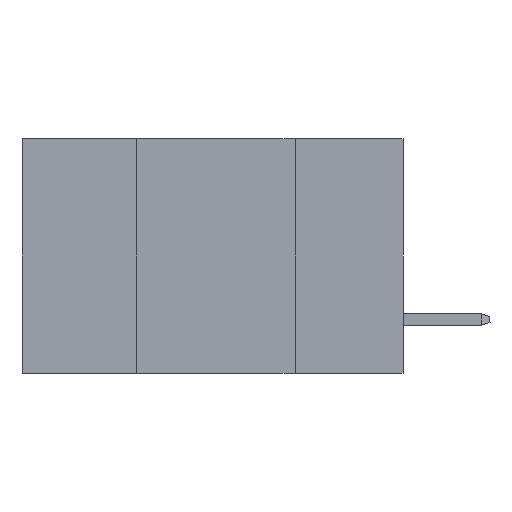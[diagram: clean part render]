
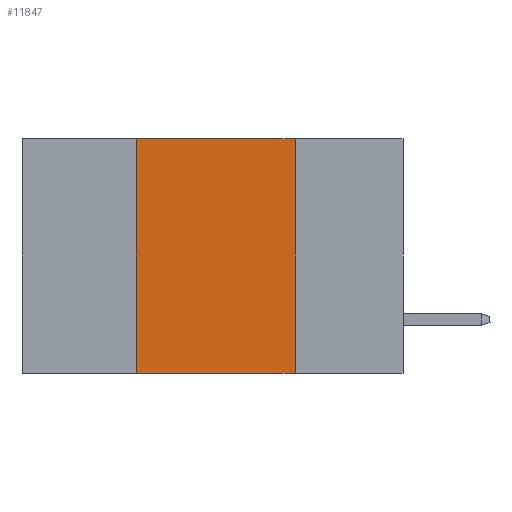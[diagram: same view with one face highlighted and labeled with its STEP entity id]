
A CAD part, left-side view. The second image highlights one B-rep face of the part: STEP entity #11847.
In plain terms, the highlighted planar face has unit normal (-1, 0, 0).
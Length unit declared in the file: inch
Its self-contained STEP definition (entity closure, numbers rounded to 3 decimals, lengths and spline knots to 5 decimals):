
#142 = DIRECTION ( 'NONE',  ( 1., 0., 0. ) ) ;
#355 = ORIENTED_EDGE ( 'NONE', *, *, #10931, .F. ) ;
#928 = EDGE_CURVE ( 'NONE', #3496, #2438, #9647, .T. ) ;
#961 = DIRECTION ( 'NONE',  ( 0., 0., -1. ) ) ;
#2438 = VERTEX_POINT ( 'NONE', #13421 ) ;
#2498 = EDGE_CURVE ( 'NONE', #3496, #14321, #9845, .T. ) ;
#3439 = DIRECTION ( 'NONE',  ( 0., 0., 1. ) ) ;
#3496 = VERTEX_POINT ( 'NONE', #16037 ) ;
#4150 = VECTOR ( 'NONE', #961, 39.37008 ) ;
#4669 = VECTOR ( 'NONE', #7395, 39.37008 ) ;
#4954 = ORIENTED_EDGE ( 'NONE', *, *, #928, .F. ) ;
#5555 = DIRECTION ( 'NONE',  ( 0., 0., -1. ) ) ;
#6455 = CARTESIAN_POINT ( 'NONE',  ( 0., 0.6, 0. ) ) ;
#7395 = DIRECTION ( 'NONE',  ( 0., -1., 0. ) ) ;
#8669 = ORIENTED_EDGE ( 'NONE', *, *, #2498, .T. ) ;
#9647 = LINE ( 'NONE', #14693, #10165 ) ;
#9770 = CARTESIAN_POINT ( 'NONE',  ( 0., 0.17, 0. ) ) ;
#9845 = LINE ( 'NONE', #13564, #4669 ) ;
#10165 = VECTOR ( 'NONE', #3439, 39.37008 ) ;
#10849 = VERTEX_POINT ( 'NONE', #11217 ) ;
#10931 = EDGE_CURVE ( 'NONE', #10849, #14321, #11530, .T. ) ;
#11022 = LINE ( 'NONE', #12100, #14716 ) ;
#11217 = CARTESIAN_POINT ( 'NONE',  ( 0., 0.17, 0. ) ) ;
#11530 = LINE ( 'NONE', #9770, #4150 ) ;
#11810 = PLANE ( 'NONE',  #12813 ) ;
#11847 = ADVANCED_FACE ( 'NONE', ( #15480 ), #11810, .F. ) ;
#12100 = CARTESIAN_POINT ( 'NONE',  ( 0., 0.6, 0. ) ) ;
#12813 = AXIS2_PLACEMENT_3D ( 'NONE', #6455, #142, #5555 ) ;
#13421 = CARTESIAN_POINT ( 'NONE',  ( 0., 0.42, 0. ) ) ;
#13564 = CARTESIAN_POINT ( 'NONE',  ( 0., 0.6, -0.37 ) ) ;
#13962 = EDGE_LOOP ( 'NONE', ( #355, #14002, #4954, #8669 ) ) ;
#14002 = ORIENTED_EDGE ( 'NONE', *, *, #16098, .F. ) ;
#14321 = VERTEX_POINT ( 'NONE', #14624 ) ;
#14610 = DIRECTION ( 'NONE',  ( 0., -1., 0. ) ) ;
#14624 = CARTESIAN_POINT ( 'NONE',  ( 0., 0.17, -0.37 ) ) ;
#14693 = CARTESIAN_POINT ( 'NONE',  ( 0., 0.42, 0. ) ) ;
#14716 = VECTOR ( 'NONE', #14610, 39.37008 ) ;
#15480 = FACE_OUTER_BOUND ( 'NONE', #13962, .T. ) ;
#16037 = CARTESIAN_POINT ( 'NONE',  ( 0., 0.42, -0.37 ) ) ;
#16098 = EDGE_CURVE ( 'NONE', #2438, #10849, #11022, .T. ) ;
